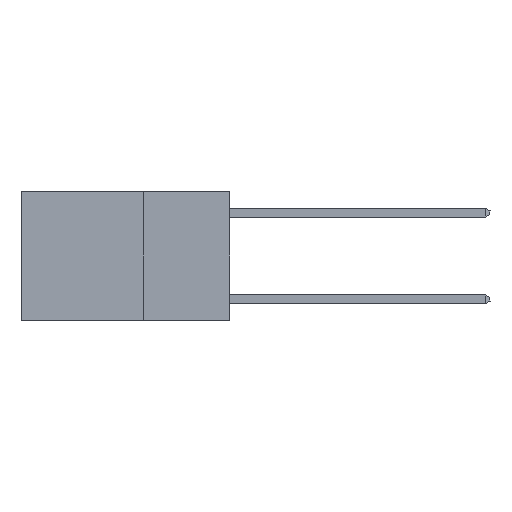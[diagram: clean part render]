
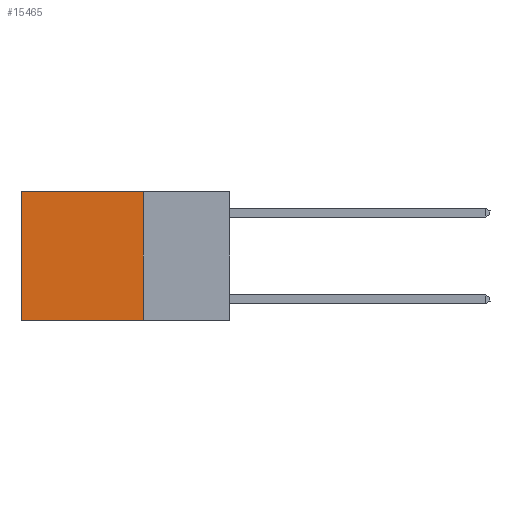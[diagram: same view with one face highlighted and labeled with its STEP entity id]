
A CAD part, left-side view. The second image highlights one B-rep face of the part: STEP entity #15465.
In plain terms, the highlighted planar face has unit normal (-1, 0, 0).
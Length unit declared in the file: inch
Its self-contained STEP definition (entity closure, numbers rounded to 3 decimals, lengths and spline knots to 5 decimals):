
#84 = CARTESIAN_POINT ( 'NONE',  ( 0.2625, 0.6, -0.37 ) ) ;
#2228 = ORIENTED_EDGE ( 'NONE', *, *, #4974, .T. ) ;
#2484 = DIRECTION ( 'NONE',  ( 1., 0., 0. ) ) ;
#2836 = ORIENTED_EDGE ( 'NONE', *, *, #6581, .F. ) ;
#3821 = VERTEX_POINT ( 'NONE', #16490 ) ;
#4135 = CARTESIAN_POINT ( 'NONE',  ( 0.2625, 0.25, 0. ) ) ;
#4263 = VERTEX_POINT ( 'NONE', #84 ) ;
#4356 = LINE ( 'NONE', #6318, #21847 ) ;
#4579 = CARTESIAN_POINT ( 'NONE',  ( 0.2625, 0.25, 0. ) ) ;
#4748 = VECTOR ( 'NONE', #11202, 39.37008 ) ;
#4974 = EDGE_CURVE ( 'NONE', #18917, #4263, #8021, .T. ) ;
#6318 = CARTESIAN_POINT ( 'NONE',  ( 0.2625, 0.25, -0.37 ) ) ;
#6581 = EDGE_CURVE ( 'NONE', #11096, #3821, #20047, .T. ) ;
#6660 = EDGE_CURVE ( 'NONE', #3821, #4263, #4356, .T. ) ;
#8021 = LINE ( 'NONE', #22220, #10998 ) ;
#9061 = ORIENTED_EDGE ( 'NONE', *, *, #12358, .T. ) ;
#9426 = FACE_OUTER_BOUND ( 'NONE', #12391, .T. ) ;
#9547 = DIRECTION ( 'NONE',  ( 0., 0., -1. ) ) ;
#9910 = DIRECTION ( 'NONE',  ( 0., 1., 0. ) ) ;
#10998 = VECTOR ( 'NONE', #15440, 39.37008 ) ;
#11096 = VERTEX_POINT ( 'NONE', #4579 ) ;
#11202 = DIRECTION ( 'NONE',  ( 0., 0., -1. ) ) ;
#12358 = EDGE_CURVE ( 'NONE', #11096, #18917, #14262, .T. ) ;
#12391 = EDGE_LOOP ( 'NONE', ( #2228, #14379, #2836, #9061 ) ) ;
#14262 = LINE ( 'NONE', #21352, #18621 ) ;
#14307 = CARTESIAN_POINT ( 'NONE',  ( 0.2625, 0.6, 0. ) ) ;
#14379 = ORIENTED_EDGE ( 'NONE', *, *, #6660, .F. ) ;
#15440 = DIRECTION ( 'NONE',  ( 0., 0., -1. ) ) ;
#15465 = ADVANCED_FACE ( 'NONE', ( #9426 ), #16521, .F. ) ;
#16490 = CARTESIAN_POINT ( 'NONE',  ( 0.2625, 0.25, -0.37 ) ) ;
#16521 = PLANE ( 'NONE',  #17170 ) ;
#17170 = AXIS2_PLACEMENT_3D ( 'NONE', #18379, #2484, #9547 ) ;
#17868 = DIRECTION ( 'NONE',  ( 0., 1., 0. ) ) ;
#18379 = CARTESIAN_POINT ( 'NONE',  ( 0.2625, 0.25, 0. ) ) ;
#18621 = VECTOR ( 'NONE', #17868, 39.37008 ) ;
#18917 = VERTEX_POINT ( 'NONE', #14307 ) ;
#20047 = LINE ( 'NONE', #4135, #4748 ) ;
#21352 = CARTESIAN_POINT ( 'NONE',  ( 0.2625, 0.25, 0. ) ) ;
#21847 = VECTOR ( 'NONE', #9910, 39.37008 ) ;
#22220 = CARTESIAN_POINT ( 'NONE',  ( 0.2625, 0.6, 0. ) ) ;
